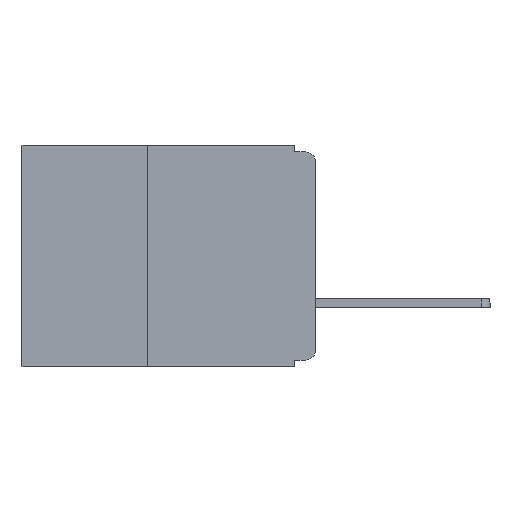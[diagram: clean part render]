
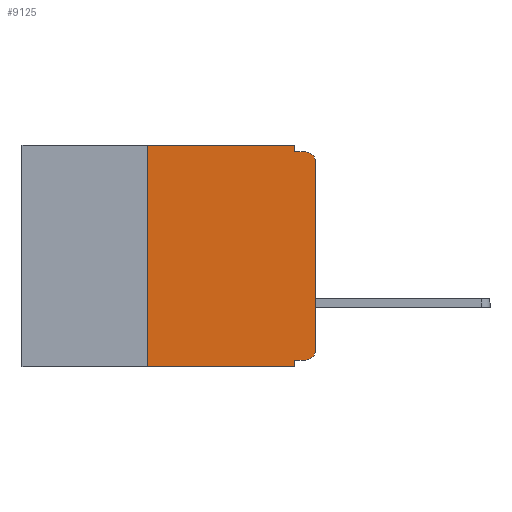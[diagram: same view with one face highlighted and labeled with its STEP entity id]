
A CAD part, left-side view. The second image highlights one B-rep face of the part: STEP entity #9125.
In plain terms, the highlighted planar face has unit normal (-1, 0, 0).
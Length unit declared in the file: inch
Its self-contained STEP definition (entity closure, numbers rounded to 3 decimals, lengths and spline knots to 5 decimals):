
#158 = VERTEX_POINT ( 'NONE', #16816 ) ;
#747 = ORIENTED_EDGE ( 'NONE', *, *, #22965, .F. ) ;
#752 = VECTOR ( 'NONE', #4345, 39.37008 ) ;
#1086 = CARTESIAN_POINT ( 'NONE',  ( 0., 0.25, 0. ) ) ;
#1691 = CARTESIAN_POINT ( 'NONE',  ( 0., 0.437, -0.33 ) ) ;
#2110 = EDGE_CURVE ( 'NONE', #7971, #24804, #14751, .T. ) ;
#2186 = CARTESIAN_POINT ( 'NONE',  ( 0., 0.031, -0.33 ) ) ;
#2456 = LINE ( 'NONE', #15396, #13741 ) ;
#2910 = FACE_OUTER_BOUND ( 'NONE', #19224, .T. ) ;
#3083 = VERTEX_POINT ( 'NONE', #12470 ) ;
#3628 = EDGE_CURVE ( 'NONE', #24804, #8516, #24920, .T. ) ;
#3730 = LINE ( 'NONE', #14902, #26791 ) ;
#3789 = DIRECTION ( 'NONE',  ( 0., 0., -1. ) ) ;
#3981 = CARTESIAN_POINT ( 'NONE',  ( 0., 0.031, 0. ) ) ;
#4295 = PLANE ( 'NONE',  #24277 ) ;
#4345 = DIRECTION ( 'NONE',  ( 0., 0., -1. ) ) ;
#4767 = VERTEX_POINT ( 'NONE', #17334 ) ;
#4835 = DIRECTION ( 'NONE',  ( 0., -1., 0. ) ) ;
#5006 = ORIENTED_EDGE ( 'NONE', *, *, #26032, .F. ) ;
#5020 = DIRECTION ( 'NONE',  ( -1., 0., 0. ) ) ;
#6026 = ORIENTED_EDGE ( 'NONE', *, *, #6938, .F. ) ;
#6595 = VERTEX_POINT ( 'NONE', #2186 ) ;
#6642 = VERTEX_POINT ( 'NONE', #28749 ) ;
#6938 = EDGE_CURVE ( 'NONE', #8363, #6642, #22293, .T. ) ;
#6994 = CARTESIAN_POINT ( 'NONE',  ( 0., 0., -0.025 ) ) ;
#7971 = VERTEX_POINT ( 'NONE', #8045 ) ;
#8045 = CARTESIAN_POINT ( 'NONE',  ( 0., 0., -0.305 ) ) ;
#8214 = EDGE_CURVE ( 'NONE', #6642, #13563, #15620, .T. ) ;
#8363 = VERTEX_POINT ( 'NONE', #1086 ) ;
#8516 = VERTEX_POINT ( 'NONE', #13409 ) ;
#8838 = DIRECTION ( 'NONE',  ( 1., 0., 0. ) ) ;
#9125 = ADVANCED_FACE ( 'NONE', ( #2910 ), #4295, .F. ) ;
#9609 = ORIENTED_EDGE ( 'NONE', *, *, #28366, .T. ) ;
#9721 = LINE ( 'NONE', #1691, #16403 ) ;
#11123 = DIRECTION ( 'NONE',  ( 0., 0., -1. ) ) ;
#11188 = DIRECTION ( 'NONE',  ( -1., 0., 0. ) ) ;
#11279 = CARTESIAN_POINT ( 'NONE',  ( 0., 0.015, -0.025 ) ) ;
#11504 = EDGE_CURVE ( 'NONE', #158, #4767, #3730, .T. ) ;
#11506 = EDGE_CURVE ( 'NONE', #3083, #6595, #9721, .T. ) ;
#12470 = CARTESIAN_POINT ( 'NONE',  ( 0., 0.25, -0.33 ) ) ;
#13277 = CARTESIAN_POINT ( 'NONE',  ( 0., 0., 0. ) ) ;
#13409 = CARTESIAN_POINT ( 'NONE',  ( 0., 0.015, -0.01 ) ) ;
#13442 = ORIENTED_EDGE ( 'NONE', *, *, #16859, .F. ) ;
#13563 = VERTEX_POINT ( 'NONE', #16149 ) ;
#13741 = VECTOR ( 'NONE', #26422, 39.37008 ) ;
#14751 = LINE ( 'NONE', #13277, #19951 ) ;
#14902 = CARTESIAN_POINT ( 'NONE',  ( 0., 0., -0.32 ) ) ;
#15091 = DIRECTION ( 'NONE',  ( 0., -1., 0. ) ) ;
#15184 = DIRECTION ( 'NONE',  ( 0., 1., 0. ) ) ;
#15396 = CARTESIAN_POINT ( 'NONE',  ( 0., 0.25, -0.33 ) ) ;
#15620 = LINE ( 'NONE', #3981, #26702 ) ;
#16042 = LINE ( 'NONE', #18253, #21961 ) ;
#16149 = CARTESIAN_POINT ( 'NONE',  ( 0., 0.031, -0.01 ) ) ;
#16369 = VECTOR ( 'NONE', #24378, 39.37008 ) ;
#16403 = VECTOR ( 'NONE', #15091, 39.37008 ) ;
#16816 = CARTESIAN_POINT ( 'NONE',  ( 0., 0.015, -0.32 ) ) ;
#16859 = EDGE_CURVE ( 'NONE', #3083, #8363, #2456, .T. ) ;
#17248 = ORIENTED_EDGE ( 'NONE', *, *, #3628, .T. ) ;
#17334 = CARTESIAN_POINT ( 'NONE',  ( 0., 0.031, -0.32 ) ) ;
#18253 = CARTESIAN_POINT ( 'NONE',  ( 0., 0., -0.01 ) ) ;
#18440 = CARTESIAN_POINT ( 'NONE',  ( 0., 0.015, -0.305 ) ) ;
#18656 = LINE ( 'NONE', #20035, #752 ) ;
#19224 = EDGE_LOOP ( 'NONE', ( #25911, #17248, #747, #20386, #6026, #13442, #22851, #5006, #27702, #9609 ) ) ;
#19951 = VECTOR ( 'NONE', #26484, 39.37008 ) ;
#20035 = CARTESIAN_POINT ( 'NONE',  ( 0., 0.031, -0.33 ) ) ;
#20386 = ORIENTED_EDGE ( 'NONE', *, *, #8214, .F. ) ;
#20484 = AXIS2_PLACEMENT_3D ( 'NONE', #18440, #5020, #20698 ) ;
#20698 = DIRECTION ( 'NONE',  ( 0., 0., -1. ) ) ;
#21961 = VECTOR ( 'NONE', #4835, 39.37008 ) ;
#22238 = CARTESIAN_POINT ( 'NONE',  ( 0., 0.437, 0. ) ) ;
#22293 = LINE ( 'NONE', #24561, #16369 ) ;
#22851 = ORIENTED_EDGE ( 'NONE', *, *, #11506, .T. ) ;
#22965 = EDGE_CURVE ( 'NONE', #13563, #8516, #16042, .T. ) ;
#23423 = CIRCLE ( 'NONE', #20484, 0.015 ) ;
#24277 = AXIS2_PLACEMENT_3D ( 'NONE', #22238, #8838, #24468 ) ;
#24378 = DIRECTION ( 'NONE',  ( 0., -1., 0. ) ) ;
#24468 = DIRECTION ( 'NONE',  ( 0., 0., -1. ) ) ;
#24561 = CARTESIAN_POINT ( 'NONE',  ( 0., 0.437, 0. ) ) ;
#24804 = VERTEX_POINT ( 'NONE', #6994 ) ;
#24920 = CIRCLE ( 'NONE', #28385, 0.015 ) ;
#25911 = ORIENTED_EDGE ( 'NONE', *, *, #2110, .T. ) ;
#26032 = EDGE_CURVE ( 'NONE', #4767, #6595, #18656, .T. ) ;
#26422 = DIRECTION ( 'NONE',  ( 0., 0., 1. ) ) ;
#26484 = DIRECTION ( 'NONE',  ( 0., 0., 1. ) ) ;
#26702 = VECTOR ( 'NONE', #3789, 39.37008 ) ;
#26791 = VECTOR ( 'NONE', #15184, 39.37008 ) ;
#27702 = ORIENTED_EDGE ( 'NONE', *, *, #11504, .F. ) ;
#28366 = EDGE_CURVE ( 'NONE', #158, #7971, #23423, .T. ) ;
#28385 = AXIS2_PLACEMENT_3D ( 'NONE', #11279, #11188, #11123 ) ;
#28749 = CARTESIAN_POINT ( 'NONE',  ( 0., 0.031, 0. ) ) ;
